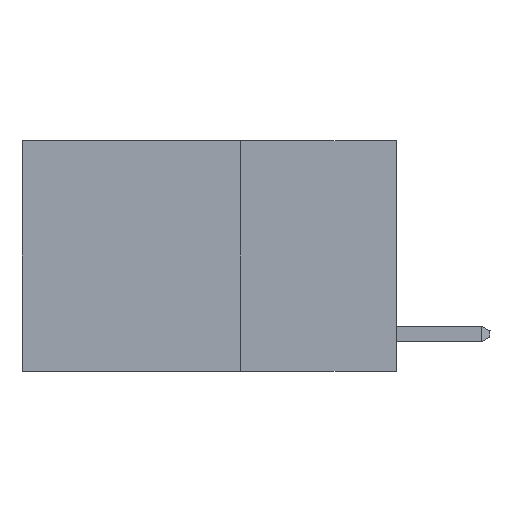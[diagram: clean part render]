
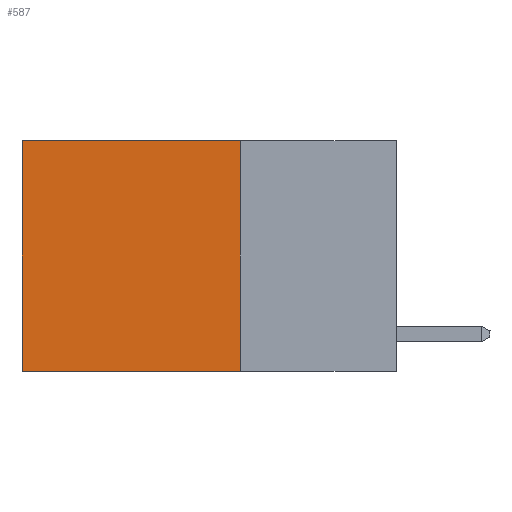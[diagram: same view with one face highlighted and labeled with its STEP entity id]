
A CAD part, left-side view. The second image highlights one B-rep face of the part: STEP entity #587.
In plain terms, the highlighted planar face has unit normal (-1, 0, 0).
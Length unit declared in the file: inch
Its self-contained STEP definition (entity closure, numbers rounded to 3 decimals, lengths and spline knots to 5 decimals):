
#127 = CARTESIAN_POINT ( 'NONE',  ( 0.2625, 0.25, 0. ) ) ;
#507 = ORIENTED_EDGE ( 'NONE', *, *, #11431, .T. ) ;
#587 = ADVANCED_FACE ( 'NONE', ( #2521 ), #11527, .F. ) ;
#1320 = DIRECTION ( 'NONE',  ( 0., 0., -1. ) ) ;
#1409 = CARTESIAN_POINT ( 'NONE',  ( 0.2625, 0.25, 0. ) ) ;
#1513 = LINE ( 'NONE', #13595, #6757 ) ;
#1984 = VERTEX_POINT ( 'NONE', #15628 ) ;
#2136 = LINE ( 'NONE', #17352, #6742 ) ;
#2209 = CARTESIAN_POINT ( 'NONE',  ( 0.2625, 0.25, -0.37 ) ) ;
#2372 = VERTEX_POINT ( 'NONE', #2209 ) ;
#2521 = FACE_OUTER_BOUND ( 'NONE', #17277, .T. ) ;
#2904 = VERTEX_POINT ( 'NONE', #14661 ) ;
#3872 = VERTEX_POINT ( 'NONE', #1409 ) ;
#5054 = VECTOR ( 'NONE', #1320, 39.37008 ) ;
#5056 = VECTOR ( 'NONE', #10661, 39.37008 ) ;
#5734 = ORIENTED_EDGE ( 'NONE', *, *, #16136, .T. ) ;
#6742 = VECTOR ( 'NONE', #17298, 39.37008 ) ;
#6757 = VECTOR ( 'NONE', #9451, 39.37008 ) ;
#7609 = DIRECTION ( 'NONE',  ( 1., 0., 0. ) ) ;
#7954 = ORIENTED_EDGE ( 'NONE', *, *, #10786, .F. ) ;
#7985 = CARTESIAN_POINT ( 'NONE',  ( 0.2625, 0.6, 0. ) ) ;
#8191 = LINE ( 'NONE', #7985, #5054 ) ;
#8962 = DIRECTION ( 'NONE',  ( 0., 0., -1. ) ) ;
#9451 = DIRECTION ( 'NONE',  ( 0., 1., 0. ) ) ;
#10661 = DIRECTION ( 'NONE',  ( 0., 1., 0. ) ) ;
#10786 = EDGE_CURVE ( 'NONE', #3872, #2372, #2136, .T. ) ;
#11431 = EDGE_CURVE ( 'NONE', #2904, #1984, #8191, .T. ) ;
#11527 = PLANE ( 'NONE',  #15467 ) ;
#12375 = LINE ( 'NONE', #127, #5056 ) ;
#13595 = CARTESIAN_POINT ( 'NONE',  ( 0.2625, 0.25, -0.37 ) ) ;
#14261 = ORIENTED_EDGE ( 'NONE', *, *, #14290, .F. ) ;
#14290 = EDGE_CURVE ( 'NONE', #2372, #1984, #1513, .T. ) ;
#14661 = CARTESIAN_POINT ( 'NONE',  ( 0.2625, 0.6, 0. ) ) ;
#15467 = AXIS2_PLACEMENT_3D ( 'NONE', #17030, #7609, #8962 ) ;
#15628 = CARTESIAN_POINT ( 'NONE',  ( 0.2625, 0.6, -0.37 ) ) ;
#16136 = EDGE_CURVE ( 'NONE', #3872, #2904, #12375, .T. ) ;
#17030 = CARTESIAN_POINT ( 'NONE',  ( 0.2625, 0.25, 0. ) ) ;
#17277 = EDGE_LOOP ( 'NONE', ( #507, #14261, #7954, #5734 ) ) ;
#17298 = DIRECTION ( 'NONE',  ( 0., 0., -1. ) ) ;
#17352 = CARTESIAN_POINT ( 'NONE',  ( 0.2625, 0.25, 0. ) ) ;
